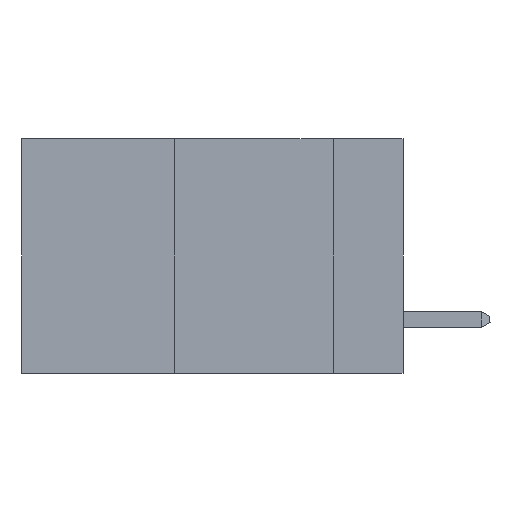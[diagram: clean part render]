
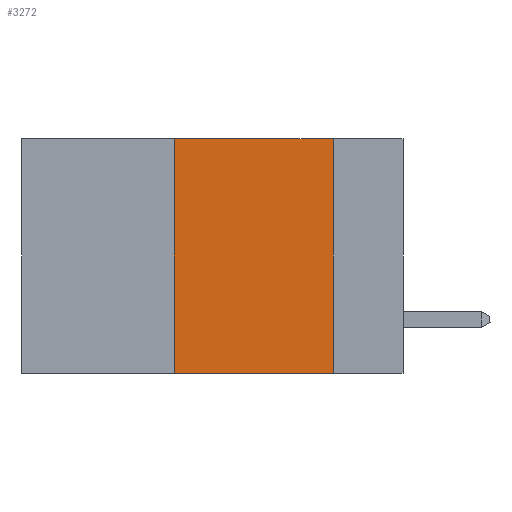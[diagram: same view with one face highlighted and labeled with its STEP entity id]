
A CAD part, left-side view. The second image highlights one B-rep face of the part: STEP entity #3272.
In plain terms, the highlighted planar face has unit normal (-1, 0, 0).
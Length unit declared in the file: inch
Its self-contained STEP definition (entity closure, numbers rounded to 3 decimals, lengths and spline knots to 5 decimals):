
#306 = CARTESIAN_POINT ( 'NONE',  ( 0., 0.6, 0. ) ) ;
#2000 = PLANE ( 'NONE',  #21141 ) ;
#2030 = DIRECTION ( 'NONE',  ( 1., 0., 0. ) ) ;
#3272 = ADVANCED_FACE ( 'NONE', ( #15044 ), #2000, .F. ) ;
#3607 = VECTOR ( 'NONE', #24907, 39.37008 ) ;
#4892 = DIRECTION ( 'NONE',  ( 0., 0., -1. ) ) ;
#5940 = EDGE_CURVE ( 'NONE', #9254, #6351, #14626, .T. ) ;
#6132 = ORIENTED_EDGE ( 'NONE', *, *, #5940, .F. ) ;
#6351 = VERTEX_POINT ( 'NONE', #22650 ) ;
#6467 = DIRECTION ( 'NONE',  ( 0., 0., 1. ) ) ;
#6931 = VERTEX_POINT ( 'NONE', #11021 ) ;
#9254 = VERTEX_POINT ( 'NONE', #22967 ) ;
#9303 = EDGE_CURVE ( 'NONE', #6351, #14319, #14090, .T. ) ;
#10904 = CARTESIAN_POINT ( 'NONE',  ( 0., 0.11, 0. ) ) ;
#11021 = CARTESIAN_POINT ( 'NONE',  ( 0., 0.36, -0.37 ) ) ;
#11644 = ORIENTED_EDGE ( 'NONE', *, *, #19980, .F. ) ;
#11837 = DIRECTION ( 'NONE',  ( 0., -1., 0. ) ) ;
#11908 = EDGE_CURVE ( 'NONE', #6931, #14319, #23495, .T. ) ;
#12642 = VECTOR ( 'NONE', #11837, 39.37008 ) ;
#13203 = EDGE_LOOP ( 'NONE', ( #25975, #6132, #11644, #22511 ) ) ;
#13858 = CARTESIAN_POINT ( 'NONE',  ( 0., 0.6, 0. ) ) ;
#14090 = LINE ( 'NONE', #10904, #23644 ) ;
#14319 = VERTEX_POINT ( 'NONE', #18213 ) ;
#14626 = LINE ( 'NONE', #13858, #3607 ) ;
#14895 = LINE ( 'NONE', #20850, #15538 ) ;
#15044 = FACE_OUTER_BOUND ( 'NONE', #13203, .T. ) ;
#15538 = VECTOR ( 'NONE', #6467, 39.37008 ) ;
#18213 = CARTESIAN_POINT ( 'NONE',  ( 0., 0.11, -0.37 ) ) ;
#19980 = EDGE_CURVE ( 'NONE', #6931, #9254, #14895, .T. ) ;
#20850 = CARTESIAN_POINT ( 'NONE',  ( 0., 0.36, 0. ) ) ;
#21141 = AXIS2_PLACEMENT_3D ( 'NONE', #306, #2030, #4892 ) ;
#22024 = CARTESIAN_POINT ( 'NONE',  ( 0., 0.6, -0.37 ) ) ;
#22511 = ORIENTED_EDGE ( 'NONE', *, *, #11908, .T. ) ;
#22650 = CARTESIAN_POINT ( 'NONE',  ( 0., 0.11, 0. ) ) ;
#22967 = CARTESIAN_POINT ( 'NONE',  ( 0., 0.36, 0. ) ) ;
#23137 = DIRECTION ( 'NONE',  ( 0., 0., -1. ) ) ;
#23495 = LINE ( 'NONE', #22024, #12642 ) ;
#23644 = VECTOR ( 'NONE', #23137, 39.37008 ) ;
#24907 = DIRECTION ( 'NONE',  ( 0., -1., 0. ) ) ;
#25975 = ORIENTED_EDGE ( 'NONE', *, *, #9303, .F. ) ;
